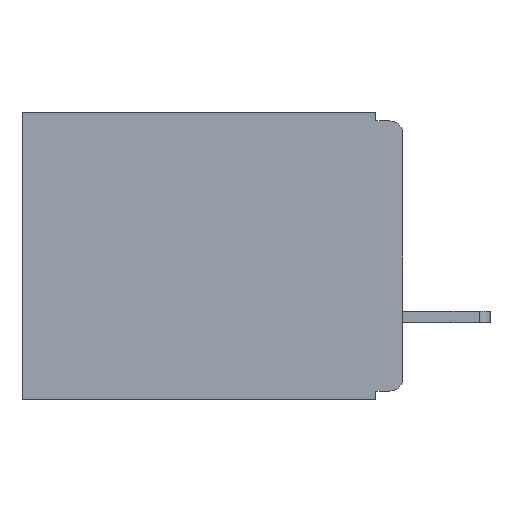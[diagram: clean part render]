
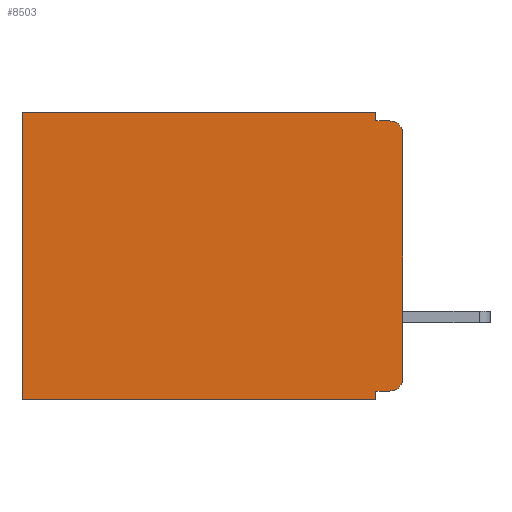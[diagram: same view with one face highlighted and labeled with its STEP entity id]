
A CAD part, left-side view. The second image highlights one B-rep face of the part: STEP entity #8503.
In plain terms, the highlighted planar face has unit normal (-1, 0, 0).
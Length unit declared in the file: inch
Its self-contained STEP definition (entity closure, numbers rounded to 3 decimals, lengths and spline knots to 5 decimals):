
#161 = DIRECTION ( 'NONE',  ( 0., 0., -1. ) ) ;
#308 = LINE ( 'NONE', #26897, #25484 ) ;
#696 = VERTEX_POINT ( 'NONE', #16368 ) ;
#1978 = VERTEX_POINT ( 'NONE', #31404 ) ;
#2515 = EDGE_CURVE ( 'NONE', #3461, #7599, #31082, .T. ) ;
#3461 = VERTEX_POINT ( 'NONE', #25048 ) ;
#3787 = CARTESIAN_POINT ( 'NONE',  ( 0.3, 0., -0.025 ) ) ;
#4021 = LINE ( 'NONE', #4573, #16328 ) ;
#4045 = VERTEX_POINT ( 'NONE', #8882 ) ;
#4573 = CARTESIAN_POINT ( 'NONE',  ( 0.3, 0.031, 0. ) ) ;
#4694 = ORIENTED_EDGE ( 'NONE', *, *, #5663, .F. ) ;
#4742 = EDGE_CURVE ( 'NONE', #29405, #696, #24289, .T. ) ;
#5434 = VECTOR ( 'NONE', #9155, 39.37008 ) ;
#5663 = EDGE_CURVE ( 'NONE', #6656, #18218, #17889, .T. ) ;
#6163 = EDGE_CURVE ( 'NONE', #1978, #20761, #4021, .T. ) ;
#6656 = VERTEX_POINT ( 'NONE', #24852 ) ;
#6753 = CARTESIAN_POINT ( 'NONE',  ( 0.3, 0.437, -0.33 ) ) ;
#6801 = DIRECTION ( 'NONE',  ( 0., 0., -1. ) ) ;
#6873 = VECTOR ( 'NONE', #12965, 39.37008 ) ;
#7025 = EDGE_CURVE ( 'NONE', #4045, #7599, #8261, .T. ) ;
#7599 = VERTEX_POINT ( 'NONE', #17445 ) ;
#7959 = DIRECTION ( 'NONE',  ( 0., 0., -1. ) ) ;
#8261 = LINE ( 'NONE', #6753, #20450 ) ;
#8503 = ADVANCED_FACE ( 'NONE', ( #26324 ), #30988, .F. ) ;
#8791 = EDGE_CURVE ( 'NONE', #20761, #696, #17313, .T. ) ;
#8882 = CARTESIAN_POINT ( 'NONE',  ( 0.3, 0.437, 0. ) ) ;
#9087 = CARTESIAN_POINT ( 'NONE',  ( 0.3, 0., -0.33 ) ) ;
#9155 = DIRECTION ( 'NONE',  ( 0., 1., 0. ) ) ;
#10031 = DIRECTION ( 'NONE',  ( -1., 0., 0. ) ) ;
#10872 = VECTOR ( 'NONE', #26264, 39.37008 ) ;
#12069 = CARTESIAN_POINT ( 'NONE',  ( 0.3, 0., -0.32 ) ) ;
#12736 = DIRECTION ( 'NONE',  ( 0., 0., -1. ) ) ;
#12926 = DIRECTION ( 'NONE',  ( 0., 1., 0. ) ) ;
#12965 = DIRECTION ( 'NONE',  ( 0., 1., 0. ) ) ;
#13295 = EDGE_CURVE ( 'NONE', #6656, #21652, #31207, .T. ) ;
#14184 = LINE ( 'NONE', #29694, #6873 ) ;
#15033 = AXIS2_PLACEMENT_3D ( 'NONE', #30915, #30762, #30651 ) ;
#15478 = EDGE_CURVE ( 'NONE', #1978, #4045, #14184, .T. ) ;
#15897 = EDGE_LOOP ( 'NONE', ( #23626, #29947, #21088, #17657, #16156, #23321, #18110, #23354, #4694, #19269 ) ) ;
#16156 = ORIENTED_EDGE ( 'NONE', *, *, #15478, .T. ) ;
#16328 = VECTOR ( 'NONE', #12736, 39.37008 ) ;
#16368 = CARTESIAN_POINT ( 'NONE',  ( 0.3, 0.015, -0.01 ) ) ;
#16546 = CARTESIAN_POINT ( 'NONE',  ( 0.3, 0.031, -0.32 ) ) ;
#17313 = LINE ( 'NONE', #26547, #10872 ) ;
#17445 = CARTESIAN_POINT ( 'NONE',  ( 0.3, 0.437, -0.33 ) ) ;
#17657 = ORIENTED_EDGE ( 'NONE', *, *, #6163, .F. ) ;
#17889 = LINE ( 'NONE', #12069, #23501 ) ;
#18109 = CARTESIAN_POINT ( 'NONE',  ( 0.3, 0.015, -0.025 ) ) ;
#18110 = ORIENTED_EDGE ( 'NONE', *, *, #2515, .F. ) ;
#18218 = VERTEX_POINT ( 'NONE', #16546 ) ;
#19239 = CARTESIAN_POINT ( 'NONE',  ( 0.3, 0.031, -0.33 ) ) ;
#19269 = ORIENTED_EDGE ( 'NONE', *, *, #13295, .T. ) ;
#19472 = VECTOR ( 'NONE', #21644, 39.37008 ) ;
#20450 = VECTOR ( 'NONE', #6801, 39.37008 ) ;
#20761 = VERTEX_POINT ( 'NONE', #22892 ) ;
#21088 = ORIENTED_EDGE ( 'NONE', *, *, #8791, .F. ) ;
#21593 = AXIS2_PLACEMENT_3D ( 'NONE', #24457, #10031, #26870 ) ;
#21644 = DIRECTION ( 'NONE',  ( 0., 0., -1. ) ) ;
#21652 = VERTEX_POINT ( 'NONE', #26998 ) ;
#22645 = EDGE_CURVE ( 'NONE', #29405, #21652, #308, .T. ) ;
#22892 = CARTESIAN_POINT ( 'NONE',  ( 0.3, 0.031, -0.01 ) ) ;
#23321 = ORIENTED_EDGE ( 'NONE', *, *, #7025, .T. ) ;
#23354 = ORIENTED_EDGE ( 'NONE', *, *, #23698, .F. ) ;
#23501 = VECTOR ( 'NONE', #12926, 39.37008 ) ;
#23626 = ORIENTED_EDGE ( 'NONE', *, *, #22645, .F. ) ;
#23698 = EDGE_CURVE ( 'NONE', #18218, #3461, #25795, .T. ) ;
#24289 = CIRCLE ( 'NONE', #27605, 0.015 ) ;
#24457 = CARTESIAN_POINT ( 'NONE',  ( 0.3, 0.015, -0.305 ) ) ;
#24852 = CARTESIAN_POINT ( 'NONE',  ( 0.3, 0.015, -0.32 ) ) ;
#25048 = CARTESIAN_POINT ( 'NONE',  ( 0.3, 0.031, -0.33 ) ) ;
#25484 = VECTOR ( 'NONE', #161, 39.37008 ) ;
#25795 = LINE ( 'NONE', #19239, #19472 ) ;
#26264 = DIRECTION ( 'NONE',  ( 0., -1., 0. ) ) ;
#26324 = FACE_OUTER_BOUND ( 'NONE', #15897, .T. ) ;
#26547 = CARTESIAN_POINT ( 'NONE',  ( 0.3, 0., -0.01 ) ) ;
#26870 = DIRECTION ( 'NONE',  ( 0., 0., -1. ) ) ;
#26897 = CARTESIAN_POINT ( 'NONE',  ( 0.3, 0., -0.33 ) ) ;
#26998 = CARTESIAN_POINT ( 'NONE',  ( 0.3, 0., -0.305 ) ) ;
#27605 = AXIS2_PLACEMENT_3D ( 'NONE', #18109, #29776, #7959 ) ;
#29405 = VERTEX_POINT ( 'NONE', #3787 ) ;
#29694 = CARTESIAN_POINT ( 'NONE',  ( 0.3, 0., 0. ) ) ;
#29776 = DIRECTION ( 'NONE',  ( -1., 0., 0. ) ) ;
#29947 = ORIENTED_EDGE ( 'NONE', *, *, #4742, .T. ) ;
#30651 = DIRECTION ( 'NONE',  ( 0., 0., -1. ) ) ;
#30762 = DIRECTION ( 'NONE',  ( 1., 0., 0. ) ) ;
#30915 = CARTESIAN_POINT ( 'NONE',  ( 0.3, 0., -0.33 ) ) ;
#30988 = PLANE ( 'NONE',  #15033 ) ;
#31082 = LINE ( 'NONE', #9087, #5434 ) ;
#31207 = CIRCLE ( 'NONE', #21593, 0.015 ) ;
#31404 = CARTESIAN_POINT ( 'NONE',  ( 0.3, 0.031, 0. ) ) ;
